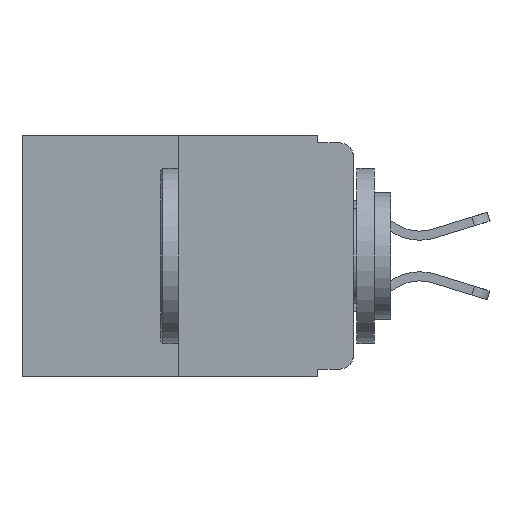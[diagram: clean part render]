
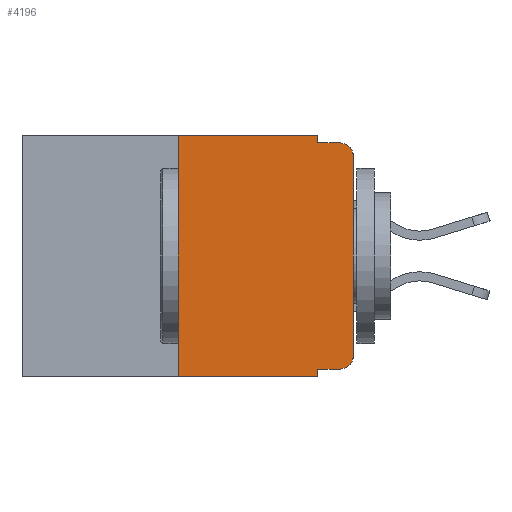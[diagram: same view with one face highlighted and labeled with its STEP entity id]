
A CAD part, left-side view. The second image highlights one B-rep face of the part: STEP entity #4196.
In plain terms, the highlighted planar face has unit normal (-1, 0, 0).
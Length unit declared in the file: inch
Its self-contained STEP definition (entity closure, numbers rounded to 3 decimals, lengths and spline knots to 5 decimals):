
#17 = VERTEX_POINT ( 'NONE', #5989 ) ;
#489 = CARTESIAN_POINT ( 'NONE',  ( 0., 0.473, 0. ) ) ;
#548 = VECTOR ( 'NONE', #25803, 39.37008 ) ;
#658 = VECTOR ( 'NONE', #22321, 39.37008 ) ;
#688 = EDGE_CURVE ( 'NONE', #3744, #895, #17040, .T. ) ;
#826 = VECTOR ( 'NONE', #9773, 39.37008 ) ;
#895 = VERTEX_POINT ( 'NONE', #24130 ) ;
#900 = DIRECTION ( 'NONE',  ( 0., 0., -1. ) ) ;
#1287 = DIRECTION ( 'NONE',  ( 1., 0., 0. ) ) ;
#1581 = EDGE_CURVE ( 'NONE', #13146, #3744, #23690, .T. ) ;
#2037 = FACE_OUTER_BOUND ( 'NONE', #11289, .T. ) ;
#2084 = ORIENTED_EDGE ( 'NONE', *, *, #7135, .T. ) ;
#2164 = EDGE_CURVE ( 'NONE', #11537, #8340, #19184, .T. ) ;
#2346 = ORIENTED_EDGE ( 'NONE', *, *, #18165, .F. ) ;
#2415 = CARTESIAN_POINT ( 'NONE',  ( 0., 0.051, 0. ) ) ;
#2624 = CARTESIAN_POINT ( 'NONE',  ( 0., 0.051, -0.333 ) ) ;
#3744 = VERTEX_POINT ( 'NONE', #13017 ) ;
#3805 = CARTESIAN_POINT ( 'NONE',  ( 0., 0.02, -0.03 ) ) ;
#4196 = ADVANCED_FACE ( 'NONE', ( #2037 ), #26391, .F. ) ;
#4248 = LINE ( 'NONE', #7630, #10342 ) ;
#4470 = AXIS2_PLACEMENT_3D ( 'NONE', #489, #1287, #900 ) ;
#4484 = DIRECTION ( 'NONE',  ( 0., -1., 0. ) ) ;
#4726 = CARTESIAN_POINT ( 'NONE',  ( 0., 0.051, 0. ) ) ;
#4735 = CARTESIAN_POINT ( 'NONE',  ( 0., 0.051, -0.333 ) ) ;
#5276 = CARTESIAN_POINT ( 'NONE',  ( 0., 0.051, -0.01 ) ) ;
#5854 = ORIENTED_EDGE ( 'NONE', *, *, #24848, .F. ) ;
#5882 = DIRECTION ( 'NONE',  ( 0., 0., -1. ) ) ;
#5989 = CARTESIAN_POINT ( 'NONE',  ( 0., 0.051, -0.343 ) ) ;
#6227 = DIRECTION ( 'NONE',  ( 0., -1., 0. ) ) ;
#6350 = LINE ( 'NONE', #15931, #826 ) ;
#6842 = ORIENTED_EDGE ( 'NONE', *, *, #20251, .F. ) ;
#6879 = CARTESIAN_POINT ( 'NONE',  ( 0., 0.02, -0.01 ) ) ;
#7135 = EDGE_CURVE ( 'NONE', #8296, #13146, #18578, .T. ) ;
#7414 = CARTESIAN_POINT ( 'NONE',  ( 0., 0.25, 0. ) ) ;
#7491 = LINE ( 'NONE', #7892, #658 ) ;
#7630 = CARTESIAN_POINT ( 'NONE',  ( 0., 0.25, 0. ) ) ;
#7703 = CARTESIAN_POINT ( 'NONE',  ( 0., 0.02, -0.333 ) ) ;
#7892 = CARTESIAN_POINT ( 'NONE',  ( 0., 0.051, 0. ) ) ;
#7973 = VECTOR ( 'NONE', #6227, 39.37008 ) ;
#8291 = CARTESIAN_POINT ( 'NONE',  ( 0., 0.473, 0. ) ) ;
#8296 = VERTEX_POINT ( 'NONE', #2624 ) ;
#8340 = VERTEX_POINT ( 'NONE', #6879 ) ;
#8468 = VERTEX_POINT ( 'NONE', #7414 ) ;
#8611 = LINE ( 'NONE', #8291, #7973 ) ;
#9177 = CARTESIAN_POINT ( 'NONE',  ( 0., 0., 0. ) ) ;
#9504 = ORIENTED_EDGE ( 'NONE', *, *, #1581, .T. ) ;
#9773 = DIRECTION ( 'NONE',  ( 0., -1., 0. ) ) ;
#9861 = EDGE_CURVE ( 'NONE', #8296, #17, #7491, .T. ) ;
#10342 = VECTOR ( 'NONE', #11659, 39.37008 ) ;
#10817 = CARTESIAN_POINT ( 'NONE',  ( 0., 0.25, -0.343 ) ) ;
#10911 = DIRECTION ( 'NONE',  ( 0., -1., 0. ) ) ;
#11113 = LINE ( 'NONE', #4726, #21392 ) ;
#11289 = EDGE_LOOP ( 'NONE', ( #18098, #19048, #14887, #5854, #6842, #2346, #24542, #20742, #2084, #9504 ) ) ;
#11537 = VERTEX_POINT ( 'NONE', #20623 ) ;
#11659 = DIRECTION ( 'NONE',  ( 0., 0., 1. ) ) ;
#12140 = VERTEX_POINT ( 'NONE', #2415 ) ;
#12370 = CIRCLE ( 'NONE', #23720, 0.02 ) ;
#13002 = DIRECTION ( 'NONE',  ( 0., 0., -1. ) ) ;
#13017 = CARTESIAN_POINT ( 'NONE',  ( 0., 0., -0.313 ) ) ;
#13091 = VECTOR ( 'NONE', #4484, 39.37008 ) ;
#13146 = VERTEX_POINT ( 'NONE', #7703 ) ;
#14887 = ORIENTED_EDGE ( 'NONE', *, *, #2164, .F. ) ;
#15931 = CARTESIAN_POINT ( 'NONE',  ( 0., 0.473, -0.343 ) ) ;
#17040 = LINE ( 'NONE', #9177, #548 ) ;
#18098 = ORIENTED_EDGE ( 'NONE', *, *, #688, .T. ) ;
#18165 = EDGE_CURVE ( 'NONE', #18499, #8468, #4248, .T. ) ;
#18216 = DIRECTION ( 'NONE',  ( -1., 0., 0. ) ) ;
#18499 = VERTEX_POINT ( 'NONE', #10817 ) ;
#18578 = LINE ( 'NONE', #4735, #22704 ) ;
#19048 = ORIENTED_EDGE ( 'NONE', *, *, #21902, .T. ) ;
#19184 = LINE ( 'NONE', #5276, #13091 ) ;
#20251 = EDGE_CURVE ( 'NONE', #8468, #12140, #8611, .T. ) ;
#20623 = CARTESIAN_POINT ( 'NONE',  ( 0., 0.051, -0.01 ) ) ;
#20674 = CARTESIAN_POINT ( 'NONE',  ( 0., 0.02, -0.313 ) ) ;
#20742 = ORIENTED_EDGE ( 'NONE', *, *, #9861, .F. ) ;
#21392 = VECTOR ( 'NONE', #13002, 39.37008 ) ;
#21902 = EDGE_CURVE ( 'NONE', #895, #8340, #12370, .T. ) ;
#22321 = DIRECTION ( 'NONE',  ( 0., 0., -1. ) ) ;
#22704 = VECTOR ( 'NONE', #10911, 39.37008 ) ;
#23690 = CIRCLE ( 'NONE', #24186, 0.02 ) ;
#23720 = AXIS2_PLACEMENT_3D ( 'NONE', #3805, #18216, #5882 ) ;
#23762 = DIRECTION ( 'NONE',  ( -1., 0., 0. ) ) ;
#23977 = EDGE_CURVE ( 'NONE', #18499, #17, #6350, .T. ) ;
#24130 = CARTESIAN_POINT ( 'NONE',  ( 0., 0., -0.03 ) ) ;
#24186 = AXIS2_PLACEMENT_3D ( 'NONE', #20674, #23762, #25419 ) ;
#24542 = ORIENTED_EDGE ( 'NONE', *, *, #23977, .T. ) ;
#24848 = EDGE_CURVE ( 'NONE', #12140, #11537, #11113, .T. ) ;
#25419 = DIRECTION ( 'NONE',  ( 0., 0., -1. ) ) ;
#25803 = DIRECTION ( 'NONE',  ( 0., 0., 1. ) ) ;
#26391 = PLANE ( 'NONE',  #4470 ) ;
